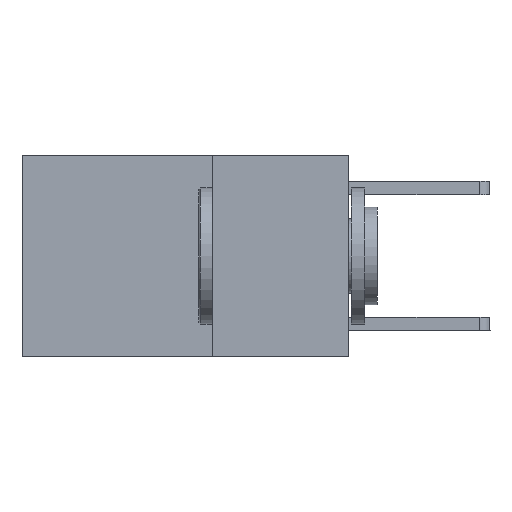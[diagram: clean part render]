
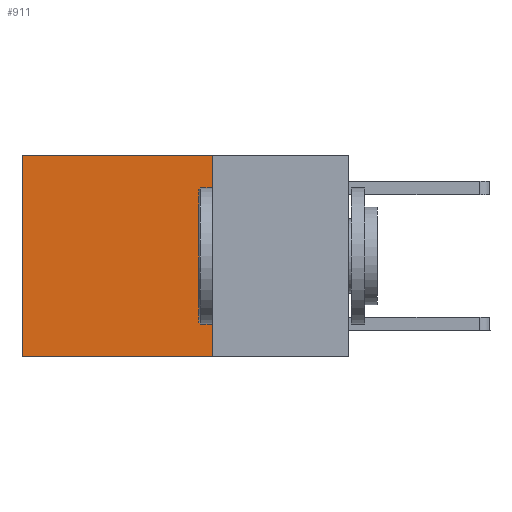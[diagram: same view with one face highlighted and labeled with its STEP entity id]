
A CAD part, left-side view. The second image highlights one B-rep face of the part: STEP entity #911.
In plain terms, the highlighted planar face has unit normal (-1, 0, 0).
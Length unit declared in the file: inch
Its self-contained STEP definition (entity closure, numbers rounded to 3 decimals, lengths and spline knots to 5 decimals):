
#189 = ORIENTED_EDGE ( 'NONE', *, *, #5540, .F. ) ;
#248 = LINE ( 'NONE', #1782, #6447 ) ;
#346 = EDGE_CURVE ( 'NONE', #5650, #6142, #9194, .T. ) ;
#450 = AXIS2_PLACEMENT_3D ( 'NONE', #1383, #9571, #7587 ) ;
#911 = ADVANCED_FACE ( 'NONE', ( #5413 ), #2886, .F. ) ;
#1383 = CARTESIAN_POINT ( 'NONE',  ( 0.2625, 0.25, 0. ) ) ;
#1606 = LINE ( 'NONE', #8245, #5390 ) ;
#1755 = LINE ( 'NONE', #3824, #5745 ) ;
#1782 = CARTESIAN_POINT ( 'NONE',  ( 0.2625, 0.25, 0. ) ) ;
#1826 = DIRECTION ( 'NONE',  ( 0., 0., -1. ) ) ;
#1919 = ORIENTED_EDGE ( 'NONE', *, *, #346, .T. ) ;
#1946 = DIRECTION ( 'NONE',  ( 0., 0., -1. ) ) ;
#2571 = ORIENTED_EDGE ( 'NONE', *, *, #7251, .T. ) ;
#2810 = CARTESIAN_POINT ( 'NONE',  ( 0.2625, 0.6, -0.37 ) ) ;
#2886 = PLANE ( 'NONE',  #450 ) ;
#2930 = VECTOR ( 'NONE', #3040, 39.37008 ) ;
#3040 = DIRECTION ( 'NONE',  ( 0., 1., 0. ) ) ;
#3357 = EDGE_CURVE ( 'NONE', #5650, #10180, #248, .T. ) ;
#3477 = VERTEX_POINT ( 'NONE', #2810 ) ;
#3824 = CARTESIAN_POINT ( 'NONE',  ( 0.2625, 0.25, -0.37 ) ) ;
#5390 = VECTOR ( 'NONE', #1946, 39.37008 ) ;
#5413 = FACE_OUTER_BOUND ( 'NONE', #9212, .T. ) ;
#5540 = EDGE_CURVE ( 'NONE', #10180, #3477, #1755, .T. ) ;
#5650 = VERTEX_POINT ( 'NONE', #6345 ) ;
#5745 = VECTOR ( 'NONE', #6989, 39.37008 ) ;
#6142 = VERTEX_POINT ( 'NONE', #9853 ) ;
#6345 = CARTESIAN_POINT ( 'NONE',  ( 0.2625, 0.25, 0. ) ) ;
#6447 = VECTOR ( 'NONE', #1826, 39.37008 ) ;
#6856 = ORIENTED_EDGE ( 'NONE', *, *, #3357, .F. ) ;
#6989 = DIRECTION ( 'NONE',  ( 0., 1., 0. ) ) ;
#7251 = EDGE_CURVE ( 'NONE', #6142, #3477, #1606, .T. ) ;
#7587 = DIRECTION ( 'NONE',  ( 0., 0., -1. ) ) ;
#8245 = CARTESIAN_POINT ( 'NONE',  ( 0.2625, 0.6, 0. ) ) ;
#9093 = CARTESIAN_POINT ( 'NONE',  ( 0.2625, 0.25, -0.37 ) ) ;
#9154 = CARTESIAN_POINT ( 'NONE',  ( 0.2625, 0.25, 0. ) ) ;
#9194 = LINE ( 'NONE', #9154, #2930 ) ;
#9212 = EDGE_LOOP ( 'NONE', ( #2571, #189, #6856, #1919 ) ) ;
#9571 = DIRECTION ( 'NONE',  ( 1., 0., 0. ) ) ;
#9853 = CARTESIAN_POINT ( 'NONE',  ( 0.2625, 0.6, 0. ) ) ;
#10180 = VERTEX_POINT ( 'NONE', #9093 ) ;
